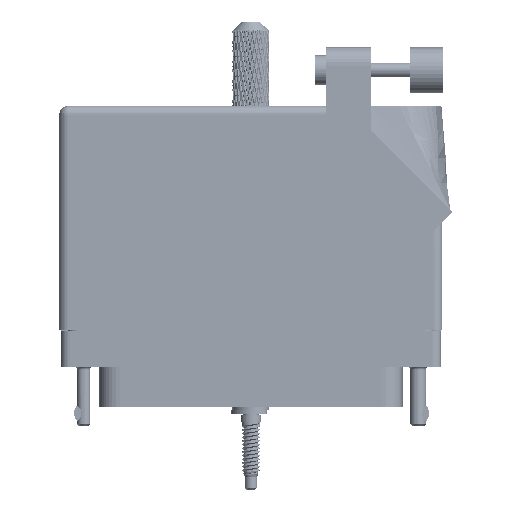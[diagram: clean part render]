
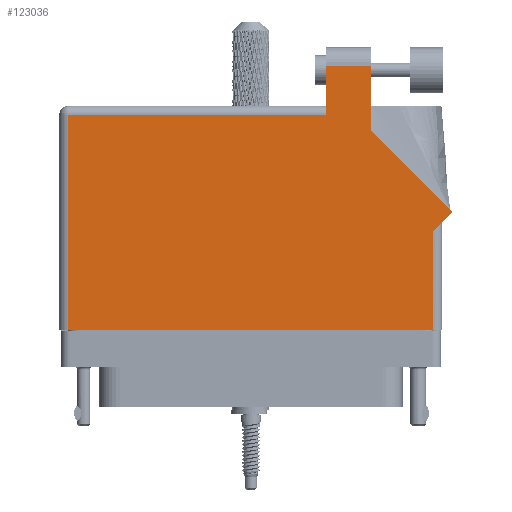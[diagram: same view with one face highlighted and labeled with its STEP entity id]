
A CAD part, front view. The second image highlights one B-rep face of the part: STEP entity #123036.
In plain terms, the highlighted face is planar.
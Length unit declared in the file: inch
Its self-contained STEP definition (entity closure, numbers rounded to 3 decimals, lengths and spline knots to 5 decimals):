
#2588 = LINE ( 'NONE', #75921, #8726 ) ;
#3166 = DIRECTION ( 'NONE',  ( 0.707, 0.707, 0. ) ) ;
#3241 = LINE ( 'NONE', #111402, #81494 ) ;
#3764 = CARTESIAN_POINT ( 'NONE',  ( 0.513, 1.705, 0.455 ) ) ;
#3982 = CARTESIAN_POINT ( 'NONE',  ( 1.306, 0.637, 0.455 ) ) ;
#5558 = ORIENTED_EDGE ( 'NONE', *, *, #56974, .T. ) ;
#5649 = LINE ( 'NONE', #6898, #82299 ) ;
#6898 = CARTESIAN_POINT ( 'NONE',  ( -1.306, -0.1, 0.455 ) ) ;
#8726 = VECTOR ( 'NONE', #55736, 39.37008 ) ;
#10419 = DIRECTION ( 'NONE',  ( -1., 0., 0. ) ) ;
#13535 = VERTEX_POINT ( 'NONE', #3764 ) ;
#13557 = LINE ( 'NONE', #116066, #33481 ) ;
#13988 = EDGE_CURVE ( 'NONE', #13535, #94186, #90125, .T. ) ;
#14031 = VERTEX_POINT ( 'NONE', #87264 ) ;
#15818 = DIRECTION ( 'NONE',  ( 0., 1., 0. ) ) ;
#26332 = ORIENTED_EDGE ( 'NONE', *, *, #123552, .T. ) ;
#30556 = DIRECTION ( 'NONE',  ( 0., 0., -1. ) ) ;
#31445 = VECTOR ( 'NONE', #3166, 39.37008 ) ;
#32170 = FACE_OUTER_BOUND ( 'NONE', #119129, .T. ) ;
#33481 = VECTOR ( 'NONE', #37322, 39.37008 ) ;
#37322 = DIRECTION ( 'NONE',  ( 0., -1., 0. ) ) ;
#37606 = EDGE_CURVE ( 'NONE', #14031, #64213, #95925, .T. ) ;
#44047 = VERTEX_POINT ( 'NONE', #82275 ) ;
#44231 = CARTESIAN_POINT ( 'NONE',  ( 1.244, 0.575, 0.455 ) ) ;
#48561 = PLANE ( 'NONE',  #61082 ) ;
#50274 = VECTOR ( 'NONE', #93641, 39.37008 ) ;
#54479 = VECTOR ( 'NONE', #15818, 39.37008 ) ;
#55116 = CARTESIAN_POINT ( 'NONE',  ( 0.513, 1.705, 0.455 ) ) ;
#55736 = DIRECTION ( 'NONE',  ( -0.707, 0.707, 0. ) ) ;
#55970 = CARTESIAN_POINT ( 'NONE',  ( 0.513, 1.43, 0.455 ) ) ;
#56974 = EDGE_CURVE ( 'NONE', #89499, #14031, #5649, .T. ) ;
#57035 = EDGE_CURVE ( 'NONE', #67450, #117200, #2588, .T. ) ;
#60392 = EDGE_CURVE ( 'NONE', #64213, #67450, #109544, .T. ) ;
#61082 = AXIS2_PLACEMENT_3D ( 'NONE', #117044, #30556, #10419 ) ;
#62008 = CARTESIAN_POINT ( 'NONE',  ( 0.513, 1.368, 0.455 ) ) ;
#62393 = CARTESIAN_POINT ( 'NONE',  ( 1.37671, 0.70771, 0.455 ) ) ;
#64213 = VERTEX_POINT ( 'NONE', #44231 ) ;
#67450 = VERTEX_POINT ( 'NONE', #62393 ) ;
#73335 = ORIENTED_EDGE ( 'NONE', *, *, #13988, .T. ) ;
#75921 = CARTESIAN_POINT ( 'NONE',  ( 1.37671, 0.70771, 0.455 ) ) ;
#77585 = CARTESIAN_POINT ( 'NONE',  ( -1.306, 1.368, 0.455 ) ) ;
#79286 = ORIENTED_EDGE ( 'NONE', *, *, #95253, .T. ) ;
#79995 = EDGE_CURVE ( 'NONE', #44047, #89499, #13557, .T. ) ;
#81494 = VECTOR ( 'NONE', #101990, 39.37008 ) ;
#82275 = CARTESIAN_POINT ( 'NONE',  ( -1.244, 1.368, 0.455 ) ) ;
#82299 = VECTOR ( 'NONE', #94276, 39.37008 ) ;
#82325 = VERTEX_POINT ( 'NONE', #90373 ) ;
#85578 = DIRECTION ( 'NONE',  ( -1., 0., 0. ) ) ;
#87264 = CARTESIAN_POINT ( 'NONE',  ( 1.244, -0.1, 0.455 ) ) ;
#89499 = VERTEX_POINT ( 'NONE', #95736 ) ;
#90125 = LINE ( 'NONE', #55970, #50274 ) ;
#90373 = CARTESIAN_POINT ( 'NONE',  ( 0.82, 1.705, 0.455 ) ) ;
#92035 = CARTESIAN_POINT ( 'NONE',  ( 1.244, 0.637, 0.455 ) ) ;
#92366 = CARTESIAN_POINT ( 'NONE',  ( 0.82, 1.26442, 0.455 ) ) ;
#93065 = ORIENTED_EDGE ( 'NONE', *, *, #60392, .T. ) ;
#93641 = DIRECTION ( 'NONE',  ( 0., -1., 0. ) ) ;
#94186 = VERTEX_POINT ( 'NONE', #62008 ) ;
#94276 = DIRECTION ( 'NONE',  ( 1., 0., 0. ) ) ;
#95253 = EDGE_CURVE ( 'NONE', #94186, #44047, #95294, .T. ) ;
#95294 = LINE ( 'NONE', #77585, #112121 ) ;
#95736 = CARTESIAN_POINT ( 'NONE',  ( -1.244, -0.1, 0.455 ) ) ;
#95925 = LINE ( 'NONE', #92035, #54479 ) ;
#97146 = ORIENTED_EDGE ( 'NONE', *, *, #57035, .T. ) ;
#97211 = DIRECTION ( 'NONE',  ( -1., 0., 0. ) ) ;
#101990 = DIRECTION ( 'NONE',  ( 0., 1., 0. ) ) ;
#107081 = ORIENTED_EDGE ( 'NONE', *, *, #112316, .T. ) ;
#107089 = LINE ( 'NONE', #55116, #120862 ) ;
#109544 = LINE ( 'NONE', #3982, #31445 ) ;
#111402 = CARTESIAN_POINT ( 'NONE',  ( 0.82, 1.26442, 0.455 ) ) ;
#112121 = VECTOR ( 'NONE', #97211, 39.37008 ) ;
#112316 = EDGE_CURVE ( 'NONE', #117200, #82325, #3241, .T. ) ;
#113655 = ORIENTED_EDGE ( 'NONE', *, *, #37606, .T. ) ;
#116066 = CARTESIAN_POINT ( 'NONE',  ( -1.244, -0.1, 0.455 ) ) ;
#117044 = CARTESIAN_POINT ( 'NONE',  ( -1.306, 1.43, 0.455 ) ) ;
#117200 = VERTEX_POINT ( 'NONE', #92366 ) ;
#119129 = EDGE_LOOP ( 'NONE', ( #107081, #26332, #73335, #79286, #125860, #5558, #113655, #93065, #97146 ) ) ;
#120862 = VECTOR ( 'NONE', #85578, 39.37008 ) ;
#123036 = ADVANCED_FACE ( 'NONE', ( #32170 ), #48561, .F. ) ;
#123552 = EDGE_CURVE ( 'NONE', #82325, #13535, #107089, .T. ) ;
#125860 = ORIENTED_EDGE ( 'NONE', *, *, #79995, .T. ) ;
